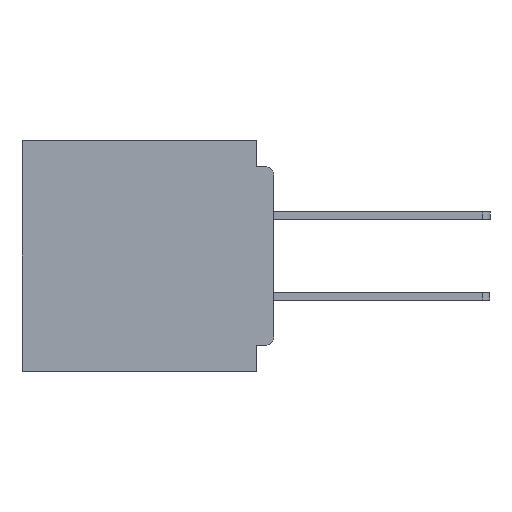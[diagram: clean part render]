
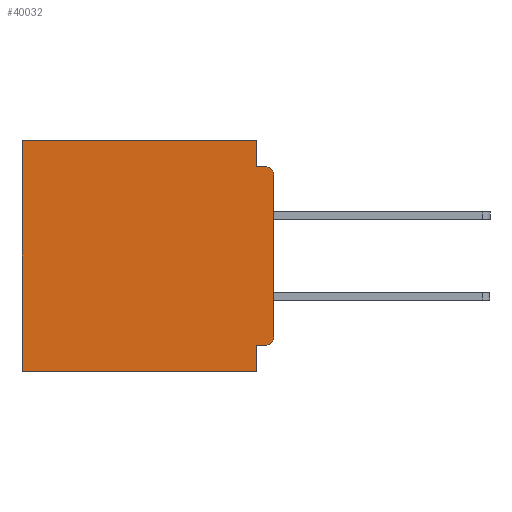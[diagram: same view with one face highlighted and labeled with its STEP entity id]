
A CAD part, left-side view. The second image highlights one B-rep face of the part: STEP entity #40032.
In plain terms, the highlighted planar face has unit normal (-1, 0, 0).
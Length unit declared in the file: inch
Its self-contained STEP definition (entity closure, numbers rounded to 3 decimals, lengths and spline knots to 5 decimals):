
#91 = CARTESIAN_POINT ( 'NONE',  ( 0.3, 0., -0.34 ) ) ;
#1091 = CARTESIAN_POINT ( 'NONE',  ( 0.3, 0., -0.4 ) ) ;
#1472 = DIRECTION ( 'NONE',  ( 0., 0., -1. ) ) ;
#2559 = VECTOR ( 'NONE', #49973, 39.37008 ) ;
#4092 = ORIENTED_EDGE ( 'NONE', *, *, #19472, .F. ) ;
#4901 = VECTOR ( 'NONE', #5332, 39.37008 ) ;
#5148 = EDGE_CURVE ( 'NONE', #46998, #15854, #53617, .T. ) ;
#5332 = DIRECTION ( 'NONE',  ( 0., 1., 0. ) ) ;
#5587 = CARTESIAN_POINT ( 'NONE',  ( 0.3, 0.437, 0. ) ) ;
#6025 = ORIENTED_EDGE ( 'NONE', *, *, #25017, .F. ) ;
#6291 = VERTEX_POINT ( 'NONE', #91 ) ;
#7088 = CARTESIAN_POINT ( 'NONE',  ( 0.3, 0., 0. ) ) ;
#8212 = DIRECTION ( 'NONE',  ( 1., 0., 0. ) ) ;
#8738 = VECTOR ( 'NONE', #44516, 39.37008 ) ;
#9011 = VERTEX_POINT ( 'NONE', #37673 ) ;
#9023 = CARTESIAN_POINT ( 'NONE',  ( 0.3, 0.015, -0.355 ) ) ;
#9252 = LINE ( 'NONE', #14888, #41085 ) ;
#9361 = CARTESIAN_POINT ( 'NONE',  ( 0.3, 0.031, 0. ) ) ;
#11306 = ORIENTED_EDGE ( 'NONE', *, *, #41452, .T. ) ;
#14888 = CARTESIAN_POINT ( 'NONE',  ( 0.3, 0.031, 0. ) ) ;
#15282 = VERTEX_POINT ( 'NONE', #41620 ) ;
#15440 = VERTEX_POINT ( 'NONE', #50923 ) ;
#15491 = VERTEX_POINT ( 'NONE', #5587 ) ;
#15776 = CARTESIAN_POINT ( 'NONE',  ( 0.3, 0., -0.4 ) ) ;
#15854 = VERTEX_POINT ( 'NONE', #20397 ) ;
#15900 = ORIENTED_EDGE ( 'NONE', *, *, #22629, .F. ) ;
#16075 = LINE ( 'NONE', #1091, #4901 ) ;
#16804 = VECTOR ( 'NONE', #1472, 39.37008 ) ;
#16815 = VERTEX_POINT ( 'NONE', #47257 ) ;
#17439 = DIRECTION ( 'NONE',  ( -1., 0., 0. ) ) ;
#19084 = DIRECTION ( 'NONE',  ( 0., 0., -1. ) ) ;
#19411 = LINE ( 'NONE', #34850, #16804 ) ;
#19472 = EDGE_CURVE ( 'NONE', #15440, #16815, #33243, .T. ) ;
#20227 = VERTEX_POINT ( 'NONE', #9361 ) ;
#20397 = CARTESIAN_POINT ( 'NONE',  ( 0.3, 0.015, -0.045 ) ) ;
#20668 = PLANE ( 'NONE',  #39839 ) ;
#21138 = CARTESIAN_POINT ( 'NONE',  ( 0.3, 0.031, -0.4 ) ) ;
#21832 = DIRECTION ( 'NONE',  ( -1., 0., 0. ) ) ;
#21989 = EDGE_CURVE ( 'NONE', #31922, #6291, #31041, .T. ) ;
#22629 = EDGE_CURVE ( 'NONE', #15282, #15854, #50909, .T. ) ;
#23978 = EDGE_CURVE ( 'NONE', #20227, #15491, #32183, .T. ) ;
#24313 = ORIENTED_EDGE ( 'NONE', *, *, #5148, .T. ) ;
#25017 = EDGE_CURVE ( 'NONE', #20227, #15282, #9252, .T. ) ;
#27780 = EDGE_CURVE ( 'NONE', #46998, #6291, #36480, .T. ) ;
#28582 = EDGE_CURVE ( 'NONE', #31922, #15440, #33152, .T. ) ;
#29281 = VECTOR ( 'NONE', #29829, 39.37008 ) ;
#29829 = DIRECTION ( 'NONE',  ( 0., 1., 0. ) ) ;
#31041 = CIRCLE ( 'NONE', #51738, 0.015 ) ;
#31922 = VERTEX_POINT ( 'NONE', #9023 ) ;
#32183 = LINE ( 'NONE', #7088, #8738 ) ;
#33151 = CARTESIAN_POINT ( 'NONE',  ( 0.3, 0., -0.4 ) ) ;
#33152 = LINE ( 'NONE', #42278, #29281 ) ;
#33243 = LINE ( 'NONE', #21138, #2559 ) ;
#34072 = ORIENTED_EDGE ( 'NONE', *, *, #27780, .F. ) ;
#34850 = CARTESIAN_POINT ( 'NONE',  ( 0.3, 0.437, -0.4 ) ) ;
#35566 = CARTESIAN_POINT ( 'NONE',  ( 0.3, 0., -0.06 ) ) ;
#36480 = LINE ( 'NONE', #15776, #44863 ) ;
#37330 = DIRECTION ( 'NONE',  ( 0., 0., -1. ) ) ;
#37673 = CARTESIAN_POINT ( 'NONE',  ( 0.3, 0.437, -0.4 ) ) ;
#39234 = ORIENTED_EDGE ( 'NONE', *, *, #23978, .T. ) ;
#39839 = AXIS2_PLACEMENT_3D ( 'NONE', #33151, #8212, #37330 ) ;
#39989 = VECTOR ( 'NONE', #52308, 39.37008 ) ;
#40032 = ADVANCED_FACE ( 'NONE', ( #52442 ), #20668, .F. ) ;
#41085 = VECTOR ( 'NONE', #19084, 39.37008 ) ;
#41452 = EDGE_CURVE ( 'NONE', #15491, #9011, #19411, .T. ) ;
#41620 = CARTESIAN_POINT ( 'NONE',  ( 0.3, 0.031, -0.045 ) ) ;
#42229 = CARTESIAN_POINT ( 'NONE',  ( 0.3, 0.015, -0.34 ) ) ;
#42278 = CARTESIAN_POINT ( 'NONE',  ( 0.3, 0., -0.355 ) ) ;
#43397 = EDGE_CURVE ( 'NONE', #16815, #9011, #16075, .T. ) ;
#44109 = CARTESIAN_POINT ( 'NONE',  ( 0.3, 0., -0.045 ) ) ;
#44516 = DIRECTION ( 'NONE',  ( 0., 1., 0. ) ) ;
#44863 = VECTOR ( 'NONE', #48824, 39.37008 ) ;
#45697 = ORIENTED_EDGE ( 'NONE', *, *, #43397, .F. ) ;
#46354 = DIRECTION ( 'NONE',  ( 0., 0., -1. ) ) ;
#46566 = CARTESIAN_POINT ( 'NONE',  ( 0.3, 0.015, -0.06 ) ) ;
#46998 = VERTEX_POINT ( 'NONE', #35566 ) ;
#47257 = CARTESIAN_POINT ( 'NONE',  ( 0.3, 0.031, -0.4 ) ) ;
#48237 = ORIENTED_EDGE ( 'NONE', *, *, #28582, .F. ) ;
#48824 = DIRECTION ( 'NONE',  ( 0., 0., -1. ) ) ;
#49513 = ORIENTED_EDGE ( 'NONE', *, *, #21989, .T. ) ;
#49973 = DIRECTION ( 'NONE',  ( 0., 0., -1. ) ) ;
#50696 = DIRECTION ( 'NONE',  ( 0., 0., -1. ) ) ;
#50909 = LINE ( 'NONE', #44109, #39989 ) ;
#50923 = CARTESIAN_POINT ( 'NONE',  ( 0.3, 0.031, -0.355 ) ) ;
#51516 = AXIS2_PLACEMENT_3D ( 'NONE', #46566, #21832, #50696 ) ;
#51738 = AXIS2_PLACEMENT_3D ( 'NONE', #42229, #17439, #46354 ) ;
#52308 = DIRECTION ( 'NONE',  ( 0., -1., 0. ) ) ;
#52442 = FACE_OUTER_BOUND ( 'NONE', #53108, .T. ) ;
#53108 = EDGE_LOOP ( 'NONE', ( #34072, #24313, #15900, #6025, #39234, #11306, #45697, #4092, #48237, #49513 ) ) ;
#53617 = CIRCLE ( 'NONE', #51516, 0.015 ) ;
